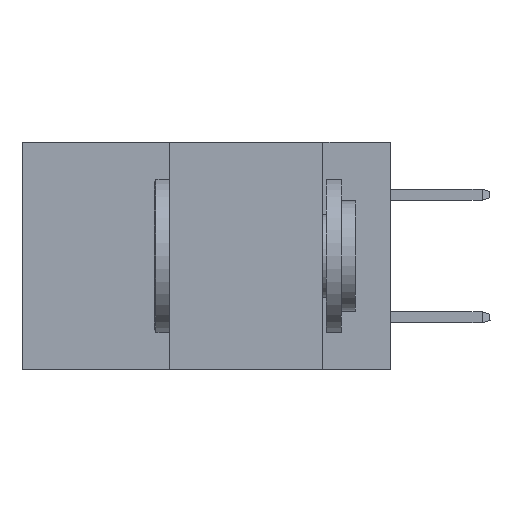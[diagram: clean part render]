
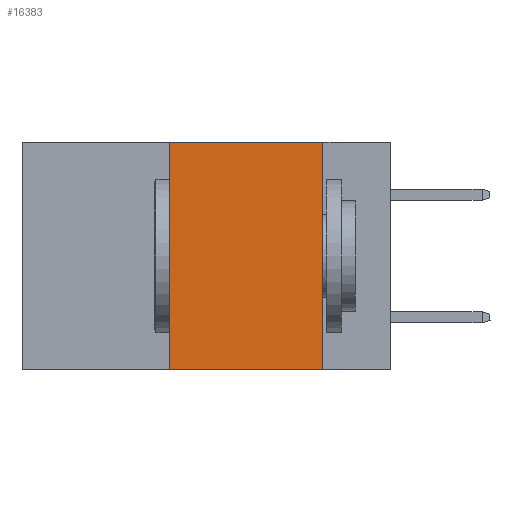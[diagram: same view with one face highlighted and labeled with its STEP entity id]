
A CAD part, left-side view. The second image highlights one B-rep face of the part: STEP entity #16383.
In plain terms, the highlighted planar face has unit normal (-1, 0, 0).
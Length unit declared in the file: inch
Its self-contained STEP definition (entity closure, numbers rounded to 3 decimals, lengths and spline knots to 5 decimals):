
#823 = CARTESIAN_POINT ( 'NONE',  ( 0., 0.6, -0.37 ) ) ;
#1296 = ORIENTED_EDGE ( 'NONE', *, *, #15342, .T. ) ;
#1386 = DIRECTION ( 'NONE',  ( 0., -1., 0. ) ) ;
#4366 = ORIENTED_EDGE ( 'NONE', *, *, #22532, .F. ) ;
#4895 = EDGE_CURVE ( 'NONE', #7117, #5151, #18239, .T. ) ;
#5043 = AXIS2_PLACEMENT_3D ( 'NONE', #16946, #6528, #18669 ) ;
#5151 = VERTEX_POINT ( 'NONE', #14645 ) ;
#5424 = VERTEX_POINT ( 'NONE', #8325 ) ;
#5600 = CARTESIAN_POINT ( 'NONE',  ( 0., 0.11, 0. ) ) ;
#6528 = DIRECTION ( 'NONE',  ( 1., 0., 0. ) ) ;
#6884 = VECTOR ( 'NONE', #18741, 39.37008 ) ;
#7117 = VERTEX_POINT ( 'NONE', #12763 ) ;
#7379 = DIRECTION ( 'NONE',  ( 0., 0., -1. ) ) ;
#8325 = CARTESIAN_POINT ( 'NONE',  ( 0., 0.11, -0.37 ) ) ;
#8804 = DIRECTION ( 'NONE',  ( 0., 0., 1. ) ) ;
#9491 = FACE_OUTER_BOUND ( 'NONE', #18060, .T. ) ;
#10723 = VECTOR ( 'NONE', #1386, 39.37008 ) ;
#11117 = EDGE_CURVE ( 'NONE', #5151, #18606, #15839, .T. ) ;
#11409 = CARTESIAN_POINT ( 'NONE',  ( 0., 0.11, 0. ) ) ;
#11788 = PLANE ( 'NONE',  #5043 ) ;
#11945 = ORIENTED_EDGE ( 'NONE', *, *, #11117, .F. ) ;
#12763 = CARTESIAN_POINT ( 'NONE',  ( 0., 0.36, -0.37 ) ) ;
#13945 = CARTESIAN_POINT ( 'NONE',  ( 0., 0.36, 0. ) ) ;
#14212 = VECTOR ( 'NONE', #8804, 39.37008 ) ;
#14645 = CARTESIAN_POINT ( 'NONE',  ( 0., 0.36, 0. ) ) ;
#14994 = VECTOR ( 'NONE', #7379, 39.37008 ) ;
#15342 = EDGE_CURVE ( 'NONE', #7117, #5424, #16703, .T. ) ;
#15839 = LINE ( 'NONE', #22250, #10723 ) ;
#16383 = ADVANCED_FACE ( 'NONE', ( #9491 ), #11788, .F. ) ;
#16703 = LINE ( 'NONE', #823, #6884 ) ;
#16946 = CARTESIAN_POINT ( 'NONE',  ( 0., 0.6, 0. ) ) ;
#18060 = EDGE_LOOP ( 'NONE', ( #4366, #11945, #18648, #1296 ) ) ;
#18239 = LINE ( 'NONE', #13945, #14212 ) ;
#18606 = VERTEX_POINT ( 'NONE', #11409 ) ;
#18648 = ORIENTED_EDGE ( 'NONE', *, *, #4895, .F. ) ;
#18669 = DIRECTION ( 'NONE',  ( 0., 0., -1. ) ) ;
#18741 = DIRECTION ( 'NONE',  ( 0., -1., 0. ) ) ;
#20012 = LINE ( 'NONE', #5600, #14994 ) ;
#22250 = CARTESIAN_POINT ( 'NONE',  ( 0., 0.6, 0. ) ) ;
#22532 = EDGE_CURVE ( 'NONE', #18606, #5424, #20012, .T. ) ;
